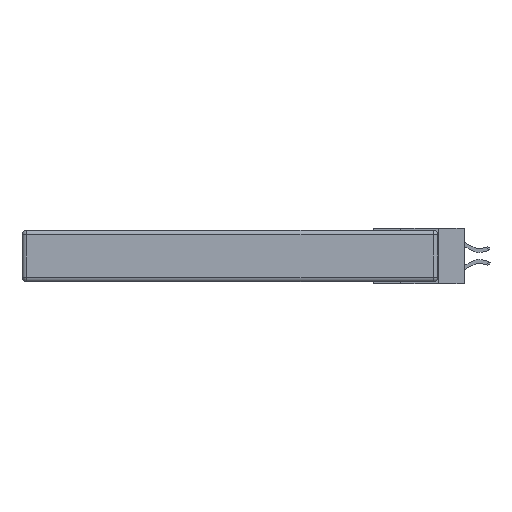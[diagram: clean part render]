
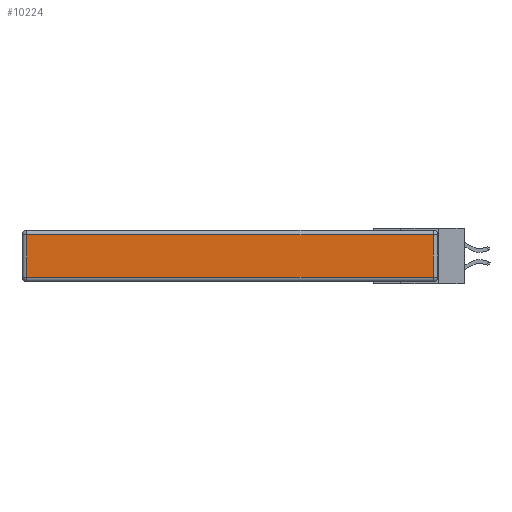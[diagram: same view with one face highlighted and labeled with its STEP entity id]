
A CAD part, left-side view. The second image highlights one B-rep face of the part: STEP entity #10224.
In plain terms, the highlighted planar face has unit normal (-1, 0, 0).
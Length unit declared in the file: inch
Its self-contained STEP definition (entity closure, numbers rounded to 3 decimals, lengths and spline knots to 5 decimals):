
#239 = DIRECTION ( 'NONE',  ( 0., 1., 0. ) ) ;
#861 = ORIENTED_EDGE ( 'NONE', *, *, #5090, .T. ) ;
#876 = CARTESIAN_POINT ( 'NONE',  ( 0., 0., -0.343 ) ) ;
#1748 = VECTOR ( 'NONE', #13315, 39.37008 ) ;
#2070 = VERTEX_POINT ( 'NONE', #14356 ) ;
#2693 = VECTOR ( 'NONE', #16627, 39.37008 ) ;
#3783 = DIRECTION ( 'NONE',  ( 0., -1., 0. ) ) ;
#3945 = VERTEX_POINT ( 'NONE', #11322 ) ;
#3949 = AXIS2_PLACEMENT_3D ( 'NONE', #876, #17198, #4941 ) ;
#3961 = VERTEX_POINT ( 'NONE', #5160 ) ;
#4424 = VECTOR ( 'NONE', #3783, 39.37008 ) ;
#4941 = DIRECTION ( 'NONE',  ( 0., 0., 1. ) ) ;
#5090 = EDGE_CURVE ( 'NONE', #17520, #2070, #8195, .T. ) ;
#5160 = CARTESIAN_POINT ( 'NONE',  ( 0., 2.72, -0.03 ) ) ;
#5709 = CARTESIAN_POINT ( 'NONE',  ( 0., 0.03, -0.313 ) ) ;
#6727 = FACE_OUTER_BOUND ( 'NONE', #11037, .T. ) ;
#7933 = ORIENTED_EDGE ( 'NONE', *, *, #8249, .T. ) ;
#7953 = CARTESIAN_POINT ( 'NONE',  ( 0., 0.03, -0.343 ) ) ;
#8195 = LINE ( 'NONE', #7953, #1748 ) ;
#8249 = EDGE_CURVE ( 'NONE', #3945, #17520, #9535, .T. ) ;
#9535 = LINE ( 'NONE', #17344, #4424 ) ;
#10012 = CARTESIAN_POINT ( 'NONE',  ( 0., 2.72, -0.343 ) ) ;
#10041 = EDGE_CURVE ( 'NONE', #2070, #3961, #15826, .T. ) ;
#10224 = ADVANCED_FACE ( 'NONE', ( #6727 ), #15844, .T. ) ;
#11037 = EDGE_LOOP ( 'NONE', ( #7933, #861, #17208, #13754 ) ) ;
#11322 = CARTESIAN_POINT ( 'NONE',  ( 0., 2.72, -0.313 ) ) ;
#11626 = VECTOR ( 'NONE', #239, 39.37008 ) ;
#12986 = LINE ( 'NONE', #10012, #2693 ) ;
#13315 = DIRECTION ( 'NONE',  ( 0., 0., 1. ) ) ;
#13754 = ORIENTED_EDGE ( 'NONE', *, *, #14009, .T. ) ;
#14009 = EDGE_CURVE ( 'NONE', #3961, #3945, #12986, .T. ) ;
#14134 = CARTESIAN_POINT ( 'NONE',  ( 0., 2.75, -0.03 ) ) ;
#14356 = CARTESIAN_POINT ( 'NONE',  ( 0., 0.03, -0.03 ) ) ;
#15826 = LINE ( 'NONE', #14134, #11626 ) ;
#15844 = PLANE ( 'NONE',  #3949 ) ;
#16627 = DIRECTION ( 'NONE',  ( 0., 0., -1. ) ) ;
#17198 = DIRECTION ( 'NONE',  ( -1., 0., 0. ) ) ;
#17208 = ORIENTED_EDGE ( 'NONE', *, *, #10041, .T. ) ;
#17344 = CARTESIAN_POINT ( 'NONE',  ( 0., 0., -0.313 ) ) ;
#17520 = VERTEX_POINT ( 'NONE', #5709 ) ;
